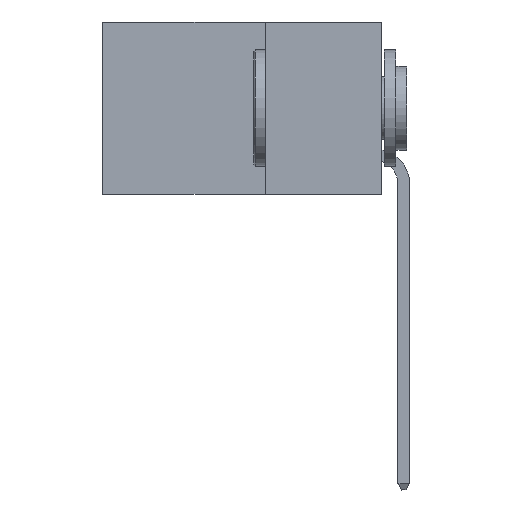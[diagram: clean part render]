
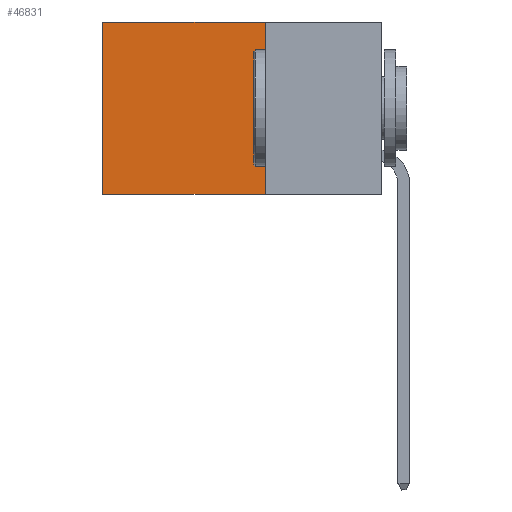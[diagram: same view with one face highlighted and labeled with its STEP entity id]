
A CAD part, left-side view. The second image highlights one B-rep face of the part: STEP entity #46831.
In plain terms, the highlighted planar face has unit normal (-1, 0, 0).
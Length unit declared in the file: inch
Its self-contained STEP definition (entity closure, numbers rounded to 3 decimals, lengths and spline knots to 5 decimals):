
#199 = AXIS2_PLACEMENT_3D ( 'NONE', #37094, #26739, #30491 ) ;
#1153 = DIRECTION ( 'NONE',  ( 0., 1., 0. ) ) ;
#1389 = DIRECTION ( 'NONE',  ( 0., 0., -1. ) ) ;
#5377 = VECTOR ( 'NONE', #6287, 39.37008 ) ;
#5559 = EDGE_CURVE ( 'NONE', #36343, #26760, #23213, .T. ) ;
#6287 = DIRECTION ( 'NONE',  ( 0., 1., 0. ) ) ;
#11311 = PLANE ( 'NONE',  #199 ) ;
#11857 = LINE ( 'NONE', #20850, #36630 ) ;
#13647 = VECTOR ( 'NONE', #1389, 39.37008 ) ;
#13777 = ORIENTED_EDGE ( 'NONE', *, *, #5559, .T. ) ;
#15775 = CARTESIAN_POINT ( 'NONE',  ( 0.2875, 0.25, 0. ) ) ;
#20053 = VERTEX_POINT ( 'NONE', #24695 ) ;
#20850 = CARTESIAN_POINT ( 'NONE',  ( 0.2875, 0.25, 0. ) ) ;
#21116 = LINE ( 'NONE', #30717, #13647 ) ;
#22769 = FACE_OUTER_BOUND ( 'NONE', #32597, .T. ) ;
#23213 = LINE ( 'NONE', #15775, #42308 ) ;
#24695 = CARTESIAN_POINT ( 'NONE',  ( 0.2875, 0.6, -0.37 ) ) ;
#25305 = EDGE_CURVE ( 'NONE', #36343, #37434, #11857, .T. ) ;
#25606 = ORIENTED_EDGE ( 'NONE', *, *, #26023, .F. ) ;
#26023 = EDGE_CURVE ( 'NONE', #37434, #20053, #44639, .T. ) ;
#26739 = DIRECTION ( 'NONE',  ( 1., 0., 0. ) ) ;
#26760 = VERTEX_POINT ( 'NONE', #47340 ) ;
#30491 = DIRECTION ( 'NONE',  ( 0., 0., -1. ) ) ;
#30717 = CARTESIAN_POINT ( 'NONE',  ( 0.2875, 0.6, 0. ) ) ;
#30845 = CARTESIAN_POINT ( 'NONE',  ( 0.2875, 0.25, 0. ) ) ;
#32597 = EDGE_LOOP ( 'NONE', ( #39111, #25606, #34120, #13777 ) ) ;
#34120 = ORIENTED_EDGE ( 'NONE', *, *, #25305, .F. ) ;
#36343 = VERTEX_POINT ( 'NONE', #30845 ) ;
#36630 = VECTOR ( 'NONE', #46661, 39.37008 ) ;
#37094 = CARTESIAN_POINT ( 'NONE',  ( 0.2875, 0.25, 0. ) ) ;
#37434 = VERTEX_POINT ( 'NONE', #41043 ) ;
#37606 = EDGE_CURVE ( 'NONE', #26760, #20053, #21116, .T. ) ;
#39111 = ORIENTED_EDGE ( 'NONE', *, *, #37606, .T. ) ;
#40129 = CARTESIAN_POINT ( 'NONE',  ( 0.2875, 0.25, -0.37 ) ) ;
#41043 = CARTESIAN_POINT ( 'NONE',  ( 0.2875, 0.25, -0.37 ) ) ;
#42308 = VECTOR ( 'NONE', #1153, 39.37008 ) ;
#44639 = LINE ( 'NONE', #40129, #5377 ) ;
#46661 = DIRECTION ( 'NONE',  ( 0., 0., -1. ) ) ;
#46831 = ADVANCED_FACE ( 'NONE', ( #22769 ), #11311, .F. ) ;
#47340 = CARTESIAN_POINT ( 'NONE',  ( 0.2875, 0.6, 0. ) ) ;
